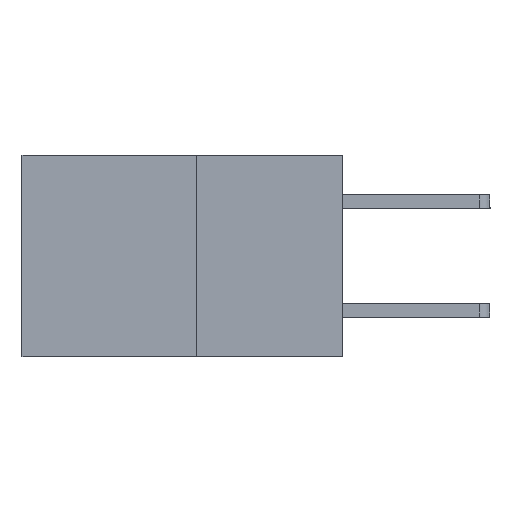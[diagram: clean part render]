
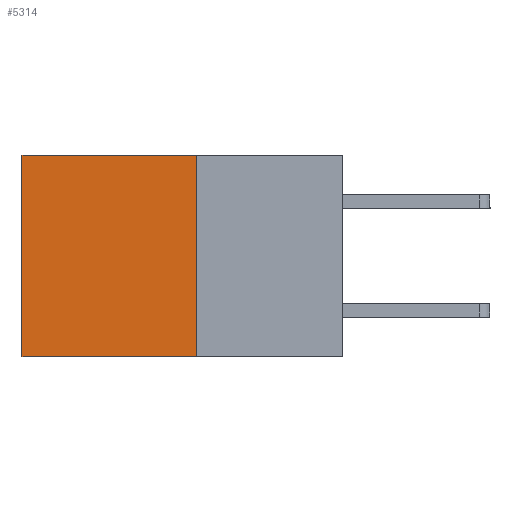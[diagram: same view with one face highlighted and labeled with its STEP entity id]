
A CAD part, left-side view. The second image highlights one B-rep face of the part: STEP entity #5314.
In plain terms, the highlighted planar face has unit normal (-1, 0, 0).
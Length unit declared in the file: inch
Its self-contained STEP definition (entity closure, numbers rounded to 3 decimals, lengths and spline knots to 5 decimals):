
#186 = CARTESIAN_POINT ( 'NONE',  ( 0.277, 0.59, 0. ) ) ;
#313 = DIRECTION ( 'NONE',  ( 0., 0., -1. ) ) ;
#703 = VERTEX_POINT ( 'NONE', #2797 ) ;
#819 = DIRECTION ( 'NONE',  ( 0., 1., 0. ) ) ;
#1281 = VECTOR ( 'NONE', #7611, 39.37008 ) ;
#1299 = LINE ( 'NONE', #3692, #8376 ) ;
#1403 = PLANE ( 'NONE',  #3538 ) ;
#1448 = CARTESIAN_POINT ( 'NONE',  ( 0.277, 0.27, -0.37 ) ) ;
#1908 = EDGE_CURVE ( 'NONE', #3487, #703, #1299, .T. ) ;
#2382 = CARTESIAN_POINT ( 'NONE',  ( 0.277, 0.27, -0.37 ) ) ;
#2797 = CARTESIAN_POINT ( 'NONE',  ( 0.277, 0.59, -0.37 ) ) ;
#2978 = VERTEX_POINT ( 'NONE', #5141 ) ;
#3070 = VECTOR ( 'NONE', #819, 39.37008 ) ;
#3487 = VERTEX_POINT ( 'NONE', #186 ) ;
#3538 = AXIS2_PLACEMENT_3D ( 'NONE', #2382, #6313, #313 ) ;
#3692 = CARTESIAN_POINT ( 'NONE',  ( 0.277, 0.59, -0.37 ) ) ;
#3714 = ORIENTED_EDGE ( 'NONE', *, *, #1908, .T. ) ;
#4432 = EDGE_CURVE ( 'NONE', #9830, #2978, #8395, .T. ) ;
#5141 = CARTESIAN_POINT ( 'NONE',  ( 0.277, 0.27, -0.37 ) ) ;
#5314 = ADVANCED_FACE ( 'NONE', ( #9398 ), #1403, .F. ) ;
#5505 = EDGE_CURVE ( 'NONE', #9830, #3487, #8655, .T. ) ;
#5636 = VECTOR ( 'NONE', #8107, 39.37008 ) ;
#5924 = CARTESIAN_POINT ( 'NONE',  ( 0.277, 0.27, -0.37 ) ) ;
#6020 = LINE ( 'NONE', #5924, #3070 ) ;
#6313 = DIRECTION ( 'NONE',  ( 1., 0., 0. ) ) ;
#6816 = EDGE_CURVE ( 'NONE', #2978, #703, #6020, .T. ) ;
#7611 = DIRECTION ( 'NONE',  ( 0., 1., 0. ) ) ;
#7682 = DIRECTION ( 'NONE',  ( 0., 0., -1. ) ) ;
#8107 = DIRECTION ( 'NONE',  ( 0., 0., -1. ) ) ;
#8376 = VECTOR ( 'NONE', #7682, 39.37008 ) ;
#8395 = LINE ( 'NONE', #1448, #5636 ) ;
#8539 = EDGE_LOOP ( 'NONE', ( #3714, #9533, #10088, #9291 ) ) ;
#8655 = LINE ( 'NONE', #10269, #1281 ) ;
#8837 = CARTESIAN_POINT ( 'NONE',  ( 0.277, 0.27, 0. ) ) ;
#9291 = ORIENTED_EDGE ( 'NONE', *, *, #5505, .T. ) ;
#9398 = FACE_OUTER_BOUND ( 'NONE', #8539, .T. ) ;
#9533 = ORIENTED_EDGE ( 'NONE', *, *, #6816, .F. ) ;
#9830 = VERTEX_POINT ( 'NONE', #8837 ) ;
#10088 = ORIENTED_EDGE ( 'NONE', *, *, #4432, .F. ) ;
#10269 = CARTESIAN_POINT ( 'NONE',  ( 0.277, 0.27, 0. ) ) ;
